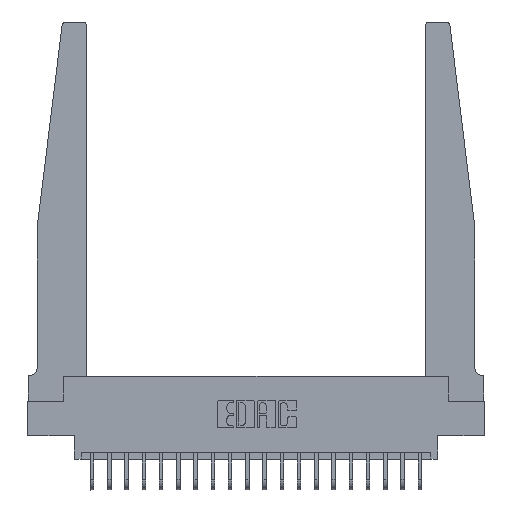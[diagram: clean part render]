
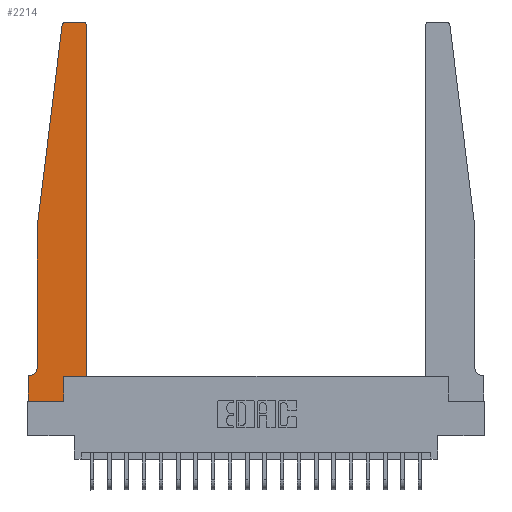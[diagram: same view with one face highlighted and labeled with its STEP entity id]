
A CAD part, top view. The second image highlights one B-rep face of the part: STEP entity #2214.
In plain terms, the highlighted planar face has unit normal (0, 0, 1).
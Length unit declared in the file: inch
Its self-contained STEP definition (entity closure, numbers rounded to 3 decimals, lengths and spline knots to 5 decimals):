
#138 = VERTEX_POINT ( 'NONE', #21719 ) ;
#469 = CARTESIAN_POINT ( 'NONE',  ( 0.065, 1.25, 0.37 ) ) ;
#747 = VERTEX_POINT ( 'NONE', #19791 ) ;
#1014 = PLANE ( 'NONE',  #14306 ) ;
#1106 = DIRECTION ( 'NONE',  ( 1., 0., 0. ) ) ;
#1215 = EDGE_CURVE ( 'NONE', #16838, #138, #17264, .T. ) ;
#1343 = CARTESIAN_POINT ( 'NONE',  ( 0., 0., 0.37 ) ) ;
#1707 = DIRECTION ( 'NONE',  ( -1., 0., 0. ) ) ;
#1807 = EDGE_CURVE ( 'NONE', #6391, #8672, #19454, .T. ) ;
#1907 = DIRECTION ( 'NONE',  ( 1., 0., 0. ) ) ;
#1951 = CARTESIAN_POINT ( 'NONE',  ( 0.27653, 2.72, 0.37 ) ) ;
#2214 = ADVANCED_FACE ( 'NONE', ( #11796 ), #1014, .T. ) ;
#2260 = ORIENTED_EDGE ( 'NONE', *, *, #19778, .T. ) ;
#2816 = VERTEX_POINT ( 'NONE', #469 ) ;
#2912 = ORIENTED_EDGE ( 'NONE', *, *, #6743, .T. ) ;
#2946 = CARTESIAN_POINT ( 'NONE',  ( 0.25, 2.75, 0.37 ) ) ;
#2961 = VECTOR ( 'NONE', #3292, 39.37008 ) ;
#3292 = DIRECTION ( 'NONE',  ( 0., 1., 0. ) ) ;
#3346 = VERTEX_POINT ( 'NONE', #21649 ) ;
#3660 = CARTESIAN_POINT ( 'NONE',  ( 0.395, 2.72, 0.37 ) ) ;
#3670 = CARTESIAN_POINT ( 'NONE',  ( 0.2605, 0.18, 0.37 ) ) ;
#4096 = VECTOR ( 'NONE', #1106, 39.37008 ) ;
#4585 = LINE ( 'NONE', #13024, #15466 ) ;
#4833 = CARTESIAN_POINT ( 'NONE',  ( 0.24675, 2.72367, 0.37 ) ) ;
#5145 = ORIENTED_EDGE ( 'NONE', *, *, #16733, .T. ) ;
#5171 = VECTOR ( 'NONE', #22300, 39.37008 ) ;
#5627 = CARTESIAN_POINT ( 'NONE',  ( 0.2605, 0., 0.37 ) ) ;
#5997 = DIRECTION ( 'NONE',  ( 0., -1., 0. ) ) ;
#6376 = LINE ( 'NONE', #1343, #4096 ) ;
#6391 = VERTEX_POINT ( 'NONE', #7054 ) ;
#6743 = EDGE_CURVE ( 'NONE', #11555, #3346, #7758, .T. ) ;
#6856 = ORIENTED_EDGE ( 'NONE', *, *, #1215, .T. ) ;
#6996 = DIRECTION ( 'NONE',  ( 1., 0., 0. ) ) ;
#7042 = ORIENTED_EDGE ( 'NONE', *, *, #10198, .T. ) ;
#7054 = CARTESIAN_POINT ( 'NONE',  ( 0., 0.1875, 0.37 ) ) ;
#7370 = CARTESIAN_POINT ( 'NONE',  ( 0.425, 2.72, 0.37 ) ) ;
#7453 = EDGE_CURVE ( 'NONE', #12645, #747, #12897, .T. ) ;
#7758 = LINE ( 'NONE', #15383, #22991 ) ;
#7767 = CARTESIAN_POINT ( 'NONE',  ( 0.2605, 0.18, 0.37 ) ) ;
#7996 = EDGE_CURVE ( 'NONE', #747, #6391, #10956, .T. ) ;
#8049 = DIRECTION ( 'NONE',  ( 0., 0., 1. ) ) ;
#8316 = LINE ( 'NONE', #15486, #14183 ) ;
#8672 = VERTEX_POINT ( 'NONE', #13474 ) ;
#10198 = EDGE_CURVE ( 'NONE', #19438, #16838, #18252, .T. ) ;
#10342 = VERTEX_POINT ( 'NONE', #4833 ) ;
#10561 = AXIS2_PLACEMENT_3D ( 'NONE', #1951, #12388, #6996 ) ;
#10684 = CARTESIAN_POINT ( 'NONE',  ( 0.425, 0.18, 0.37 ) ) ;
#10810 = VERTEX_POINT ( 'NONE', #5627 ) ;
#10847 = CARTESIAN_POINT ( 'NONE',  ( 0.065, 0.1875, 0.37 ) ) ;
#10956 = LINE ( 'NONE', #10847, #14796 ) ;
#10971 = ORIENTED_EDGE ( 'NONE', *, *, #7453, .T. ) ;
#10988 = DIRECTION ( 'NONE',  ( 0., 0., -1. ) ) ;
#11555 = VERTEX_POINT ( 'NONE', #7767 ) ;
#11608 = ORIENTED_EDGE ( 'NONE', *, *, #21091, .T. ) ;
#11796 = FACE_OUTER_BOUND ( 'NONE', #13288, .T. ) ;
#12040 = VECTOR ( 'NONE', #12063, 39.37008 ) ;
#12063 = DIRECTION ( 'NONE',  ( 0., -1., 0. ) ) ;
#12388 = DIRECTION ( 'NONE',  ( 0., 0., 1. ) ) ;
#12471 = LINE ( 'NONE', #3670, #15073 ) ;
#12612 = CARTESIAN_POINT ( 'NONE',  ( 0.065, 0.2375, 0.37 ) ) ;
#12645 = VERTEX_POINT ( 'NONE', #12612 ) ;
#12897 = CIRCLE ( 'NONE', #19673, 0.05 ) ;
#13024 = CARTESIAN_POINT ( 'NONE',  ( 0.065, 1.25, 0.37 ) ) ;
#13142 = DIRECTION ( 'NONE',  ( 1., 0., 0. ) ) ;
#13257 = ORIENTED_EDGE ( 'NONE', *, *, #7996, .T. ) ;
#13288 = EDGE_LOOP ( 'NONE', ( #6856, #2260, #5145, #13451, #10971, #13257, #21951, #22767, #11608, #2912, #19305, #7042 ) ) ;
#13451 = ORIENTED_EDGE ( 'NONE', *, *, #22968, .T. ) ;
#13474 = CARTESIAN_POINT ( 'NONE',  ( 0., 0., 0.37 ) ) ;
#13556 = CARTESIAN_POINT ( 'NONE',  ( 0., 0.1875, 0.37 ) ) ;
#14183 = VECTOR ( 'NONE', #20869, 39.37008 ) ;
#14227 = DIRECTION ( 'NONE',  ( 0., 1., 0. ) ) ;
#14242 = EDGE_CURVE ( 'NONE', #3346, #19438, #15739, .T. ) ;
#14306 = AXIS2_PLACEMENT_3D ( 'NONE', #13556, #8049, #22355 ) ;
#14502 = DIRECTION ( 'NONE',  ( -1., 0., 0. ) ) ;
#14770 = EDGE_CURVE ( 'NONE', #8672, #10810, #6376, .T. ) ;
#14796 = VECTOR ( 'NONE', #1707, 39.37008 ) ;
#14810 = AXIS2_PLACEMENT_3D ( 'NONE', #3660, #17990, #1907 ) ;
#15073 = VECTOR ( 'NONE', #14227, 39.37008 ) ;
#15383 = CARTESIAN_POINT ( 'NONE',  ( 0.425, 0.18, 0.37 ) ) ;
#15466 = VECTOR ( 'NONE', #5997, 39.37008 ) ;
#15486 = CARTESIAN_POINT ( 'NONE',  ( 0.065, 1.25, 0.37 ) ) ;
#15739 = LINE ( 'NONE', #10684, #2961 ) ;
#16733 = EDGE_CURVE ( 'NONE', #10342, #2816, #8316, .T. ) ;
#16838 = VERTEX_POINT ( 'NONE', #17819 ) ;
#17264 = LINE ( 'NONE', #2946, #5171 ) ;
#17819 = CARTESIAN_POINT ( 'NONE',  ( 0.395, 2.75, 0.37 ) ) ;
#17990 = DIRECTION ( 'NONE',  ( 0., 0., 1. ) ) ;
#18252 = CIRCLE ( 'NONE', #14810, 0.03 ) ;
#18278 = CARTESIAN_POINT ( 'NONE',  ( 0.015, 0.2375, 0.37 ) ) ;
#19305 = ORIENTED_EDGE ( 'NONE', *, *, #14242, .T. ) ;
#19438 = VERTEX_POINT ( 'NONE', #7370 ) ;
#19454 = LINE ( 'NONE', #23060, #12040 ) ;
#19673 = AXIS2_PLACEMENT_3D ( 'NONE', #18278, #10988, #14502 ) ;
#19778 = EDGE_CURVE ( 'NONE', #138, #10342, #20277, .T. ) ;
#19791 = CARTESIAN_POINT ( 'NONE',  ( 0.015, 0.1875, 0.37 ) ) ;
#20277 = CIRCLE ( 'NONE', #10561, 0.03 ) ;
#20869 = DIRECTION ( 'NONE',  ( -0.122, -0.992, 0. ) ) ;
#21091 = EDGE_CURVE ( 'NONE', #10810, #11555, #12471, .T. ) ;
#21649 = CARTESIAN_POINT ( 'NONE',  ( 0.425, 0.18, 0.37 ) ) ;
#21719 = CARTESIAN_POINT ( 'NONE',  ( 0.27653, 2.75, 0.37 ) ) ;
#21951 = ORIENTED_EDGE ( 'NONE', *, *, #1807, .T. ) ;
#22300 = DIRECTION ( 'NONE',  ( -1., 0., 0. ) ) ;
#22355 = DIRECTION ( 'NONE',  ( 1., 0., 0. ) ) ;
#22767 = ORIENTED_EDGE ( 'NONE', *, *, #14770, .T. ) ;
#22968 = EDGE_CURVE ( 'NONE', #2816, #12645, #4585, .T. ) ;
#22991 = VECTOR ( 'NONE', #13142, 39.37008 ) ;
#23060 = CARTESIAN_POINT ( 'NONE',  ( 0., 0., 0.37 ) ) ;
